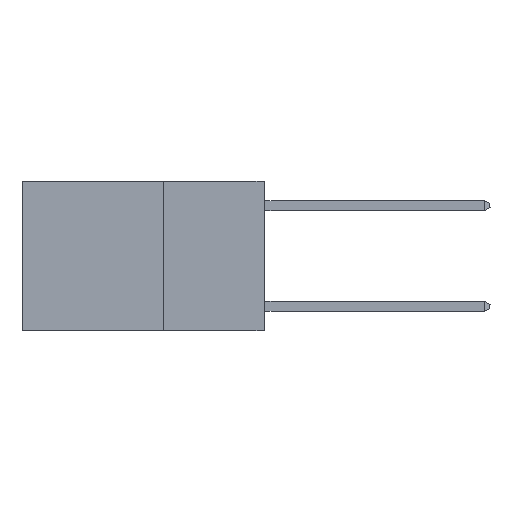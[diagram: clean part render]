
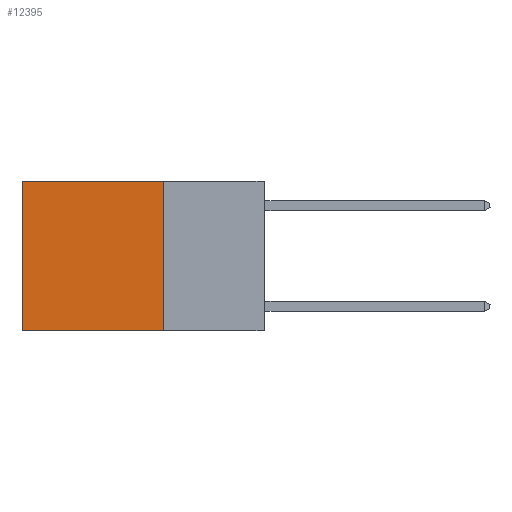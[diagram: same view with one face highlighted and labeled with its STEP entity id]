
A CAD part, left-side view. The second image highlights one B-rep face of the part: STEP entity #12395.
In plain terms, the highlighted planar face has unit normal (-1, 0, 0).
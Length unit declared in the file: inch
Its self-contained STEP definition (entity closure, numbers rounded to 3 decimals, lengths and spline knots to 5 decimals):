
#234 = CARTESIAN_POINT ( 'NONE',  ( 0.2625, 0.25, 0. ) ) ;
#1136 = EDGE_CURVE ( 'NONE', #19633, #19003, #25771, .T. ) ;
#1976 = CARTESIAN_POINT ( 'NONE',  ( 0.2625, 0.25, -0.37 ) ) ;
#3076 = EDGE_CURVE ( 'NONE', #27005, #19633, #3163, .T. ) ;
#3163 = LINE ( 'NONE', #11717, #11541 ) ;
#3276 = EDGE_CURVE ( 'NONE', #27005, #8306, #23436, .T. ) ;
#3939 = CARTESIAN_POINT ( 'NONE',  ( 0.2625, 0.6, -0.37 ) ) ;
#4700 = PLANE ( 'NONE',  #12380 ) ;
#5941 = ORIENTED_EDGE ( 'NONE', *, *, #13947, .T. ) ;
#6541 = CARTESIAN_POINT ( 'NONE',  ( 0.2625, 0.25, -0.37 ) ) ;
#6842 = ORIENTED_EDGE ( 'NONE', *, *, #3076, .F. ) ;
#8123 = ORIENTED_EDGE ( 'NONE', *, *, #3276, .T. ) ;
#8306 = VERTEX_POINT ( 'NONE', #13622 ) ;
#8766 = DIRECTION ( 'NONE',  ( 0., 0., -1. ) ) ;
#10677 = EDGE_LOOP ( 'NONE', ( #5941, #26087, #6842, #8123 ) ) ;
#10768 = CARTESIAN_POINT ( 'NONE',  ( 0.2625, 0.25, 0. ) ) ;
#11541 = VECTOR ( 'NONE', #14179, 39.37008 ) ;
#11717 = CARTESIAN_POINT ( 'NONE',  ( 0.2625, 0.25, 0. ) ) ;
#12380 = AXIS2_PLACEMENT_3D ( 'NONE', #10768, #13085, #8766 ) ;
#12395 = ADVANCED_FACE ( 'NONE', ( #15699 ), #4700, .F. ) ;
#12425 = CARTESIAN_POINT ( 'NONE',  ( 0.2625, 0.25, 0. ) ) ;
#13082 = VECTOR ( 'NONE', #15181, 39.37008 ) ;
#13085 = DIRECTION ( 'NONE',  ( 1., 0., 0. ) ) ;
#13622 = CARTESIAN_POINT ( 'NONE',  ( 0.2625, 0.6, 0. ) ) ;
#13947 = EDGE_CURVE ( 'NONE', #8306, #19003, #13968, .T. ) ;
#13968 = LINE ( 'NONE', #22957, #25860 ) ;
#14179 = DIRECTION ( 'NONE',  ( 0., 0., -1. ) ) ;
#15181 = DIRECTION ( 'NONE',  ( 0., 1., 0. ) ) ;
#15699 = FACE_OUTER_BOUND ( 'NONE', #10677, .T. ) ;
#19003 = VERTEX_POINT ( 'NONE', #3939 ) ;
#19510 = DIRECTION ( 'NONE',  ( 0., 1., 0. ) ) ;
#19633 = VERTEX_POINT ( 'NONE', #6541 ) ;
#22957 = CARTESIAN_POINT ( 'NONE',  ( 0.2625, 0.6, 0. ) ) ;
#23436 = LINE ( 'NONE', #12425, #25005 ) ;
#25005 = VECTOR ( 'NONE', #19510, 39.37008 ) ;
#25411 = DIRECTION ( 'NONE',  ( 0., 0., -1. ) ) ;
#25771 = LINE ( 'NONE', #1976, #13082 ) ;
#25860 = VECTOR ( 'NONE', #25411, 39.37008 ) ;
#26087 = ORIENTED_EDGE ( 'NONE', *, *, #1136, .F. ) ;
#27005 = VERTEX_POINT ( 'NONE', #234 ) ;
